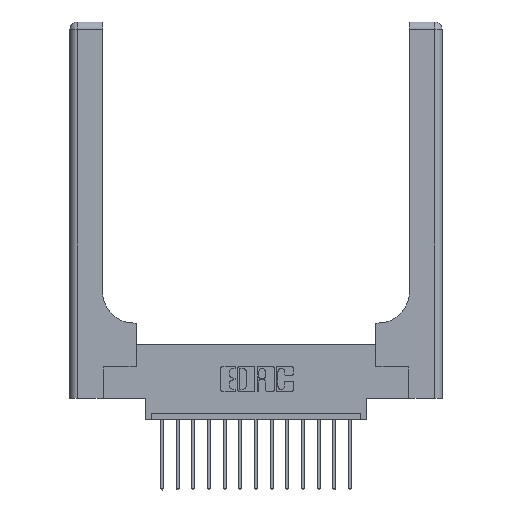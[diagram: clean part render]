
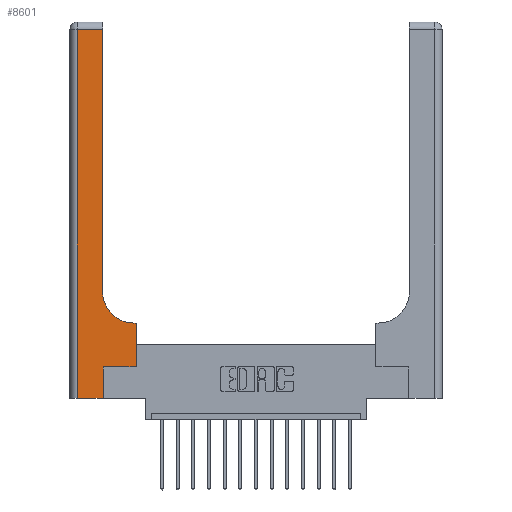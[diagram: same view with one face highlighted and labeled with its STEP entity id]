
A CAD part, top view. The second image highlights one B-rep face of the part: STEP entity #8601.
In plain terms, the highlighted planar face has unit normal (0, 0, 1).
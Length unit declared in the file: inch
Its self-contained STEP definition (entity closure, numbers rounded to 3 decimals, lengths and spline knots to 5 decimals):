
#42 = EDGE_CURVE ( 'NONE', #6891, #10565, #13729, .T. ) ;
#157 = DIRECTION ( 'NONE',  ( 0., 0., -1. ) ) ;
#369 = ORIENTED_EDGE ( 'NONE', *, *, #501, .T. ) ;
#501 = EDGE_CURVE ( 'NONE', #4503, #6237, #9747, .T. ) ;
#733 = VECTOR ( 'NONE', #14836, 39.37008 ) ;
#774 = ORIENTED_EDGE ( 'NONE', *, *, #1251, .T. ) ;
#927 = EDGE_CURVE ( 'NONE', #17164, #3581, #6775, .T. ) ;
#1078 = ORIENTED_EDGE ( 'NONE', *, *, #42, .T. ) ;
#1251 = EDGE_CURVE ( 'NONE', #12121, #12830, #13312, .T. ) ;
#1314 = CARTESIAN_POINT ( 'NONE',  ( 0.528, 0.25, 0.37 ) ) ;
#1392 = PLANE ( 'NONE',  #4247 ) ;
#1397 = VECTOR ( 'NONE', #10640, 39.37008 ) ;
#1515 = CARTESIAN_POINT ( 'NONE',  ( 0.265, 0.25, 0.37 ) ) ;
#1680 = ORIENTED_EDGE ( 'NONE', *, *, #5093, .T. ) ;
#1954 = CARTESIAN_POINT ( 'NONE',  ( 0.06, 2.94, 0.37 ) ) ;
#2402 = CARTESIAN_POINT ( 'NONE',  ( 0.26, 0.85, 0.37 ) ) ;
#2802 = DIRECTION ( 'NONE',  ( -1., 0., 0. ) ) ;
#3148 = EDGE_CURVE ( 'NONE', #6237, #6891, #13888, .T. ) ;
#3446 = DIRECTION ( 'NONE',  ( 0., 0., -1. ) ) ;
#3504 = DIRECTION ( 'NONE',  ( 1., 0., 0. ) ) ;
#3558 = CARTESIAN_POINT ( 'NONE',  ( 0.265, 0., 0.37 ) ) ;
#3581 = VERTEX_POINT ( 'NONE', #1954 ) ;
#3751 = EDGE_LOOP ( 'NONE', ( #1680, #9138, #16875, #369, #9006, #1078, #6768, #8202, #774 ) ) ;
#3801 = DIRECTION ( 'NONE',  ( 1., 0., 0. ) ) ;
#4036 = CARTESIAN_POINT ( 'NONE',  ( 0.51, 0.6, 0.37 ) ) ;
#4229 = EDGE_CURVE ( 'NONE', #10565, #9598, #17049, .T. ) ;
#4247 = AXIS2_PLACEMENT_3D ( 'NONE', #8127, #157, #2802 ) ;
#4461 = CARTESIAN_POINT ( 'NONE',  ( 0.06, 0., 0.37 ) ) ;
#4503 = VERTEX_POINT ( 'NONE', #4461 ) ;
#4675 = LINE ( 'NONE', #11919, #6336 ) ;
#4715 = CARTESIAN_POINT ( 'NONE',  ( 0., 2.94, 0.37 ) ) ;
#4919 = VECTOR ( 'NONE', #10253, 39.37008 ) ;
#5093 = EDGE_CURVE ( 'NONE', #12830, #17164, #6352, .T. ) ;
#5373 = DIRECTION ( 'NONE',  ( 0., -1., 0. ) ) ;
#5497 = EDGE_CURVE ( 'NONE', #3581, #4503, #4675, .T. ) ;
#6237 = VERTEX_POINT ( 'NONE', #16828 ) ;
#6257 = CARTESIAN_POINT ( 'NONE',  ( 0.26, 0.6, 0.37 ) ) ;
#6336 = VECTOR ( 'NONE', #5373, 39.37008 ) ;
#6352 = LINE ( 'NONE', #12120, #733 ) ;
#6768 = ORIENTED_EDGE ( 'NONE', *, *, #4229, .T. ) ;
#6775 = LINE ( 'NONE', #4715, #4919 ) ;
#6891 = VERTEX_POINT ( 'NONE', #11469 ) ;
#7269 = FACE_OUTER_BOUND ( 'NONE', #3751, .T. ) ;
#8127 = CARTESIAN_POINT ( 'NONE',  ( 0., 3., 0.37 ) ) ;
#8202 = ORIENTED_EDGE ( 'NONE', *, *, #14473, .T. ) ;
#8601 = ADVANCED_FACE ( 'NONE', ( #7269 ), #1392, .F. ) ;
#8909 = DIRECTION ( 'NONE',  ( 0., 1., 0. ) ) ;
#9006 = ORIENTED_EDGE ( 'NONE', *, *, #3148, .T. ) ;
#9138 = ORIENTED_EDGE ( 'NONE', *, *, #927, .T. ) ;
#9156 = CARTESIAN_POINT ( 'NONE',  ( 0., 0., 0.37 ) ) ;
#9356 = VECTOR ( 'NONE', #15655, 39.37008 ) ;
#9515 = VECTOR ( 'NONE', #11343, 39.37008 ) ;
#9598 = VERTEX_POINT ( 'NONE', #15862 ) ;
#9747 = LINE ( 'NONE', #9156, #15413 ) ;
#10173 = CARTESIAN_POINT ( 'NONE',  ( 0.528, 0.25, 0.37 ) ) ;
#10253 = DIRECTION ( 'NONE',  ( -1., 0., 0. ) ) ;
#10565 = VERTEX_POINT ( 'NONE', #10173 ) ;
#10640 = DIRECTION ( 'NONE',  ( 0., 1., 0. ) ) ;
#10994 = VECTOR ( 'NONE', #8909, 39.37008 ) ;
#11343 = DIRECTION ( 'NONE',  ( 1., 0., 0. ) ) ;
#11382 = CARTESIAN_POINT ( 'NONE',  ( 0.51, 0.85, 0.37 ) ) ;
#11469 = CARTESIAN_POINT ( 'NONE',  ( 0.265, 0.25, 0.37 ) ) ;
#11919 = CARTESIAN_POINT ( 'NONE',  ( 0.06, 3., 0.37 ) ) ;
#12120 = CARTESIAN_POINT ( 'NONE',  ( 0.26, 3., 0.37 ) ) ;
#12121 = VERTEX_POINT ( 'NONE', #4036 ) ;
#12830 = VERTEX_POINT ( 'NONE', #2402 ) ;
#13312 = CIRCLE ( 'NONE', #16197, 0.25 ) ;
#13729 = LINE ( 'NONE', #1515, #9515 ) ;
#13888 = LINE ( 'NONE', #3558, #10994 ) ;
#14473 = EDGE_CURVE ( 'NONE', #9598, #12121, #14826, .T. ) ;
#14826 = LINE ( 'NONE', #6257, #9356 ) ;
#14836 = DIRECTION ( 'NONE',  ( 0., 1., 0. ) ) ;
#15403 = CARTESIAN_POINT ( 'NONE',  ( 0.26, 2.94, 0.37 ) ) ;
#15413 = VECTOR ( 'NONE', #3801, 39.37008 ) ;
#15655 = DIRECTION ( 'NONE',  ( -1., 0., 0. ) ) ;
#15862 = CARTESIAN_POINT ( 'NONE',  ( 0.528, 0.6, 0.37 ) ) ;
#16197 = AXIS2_PLACEMENT_3D ( 'NONE', #11382, #3446, #3504 ) ;
#16828 = CARTESIAN_POINT ( 'NONE',  ( 0.265, 0., 0.37 ) ) ;
#16875 = ORIENTED_EDGE ( 'NONE', *, *, #5497, .T. ) ;
#17049 = LINE ( 'NONE', #1314, #1397 ) ;
#17164 = VERTEX_POINT ( 'NONE', #15403 ) ;
